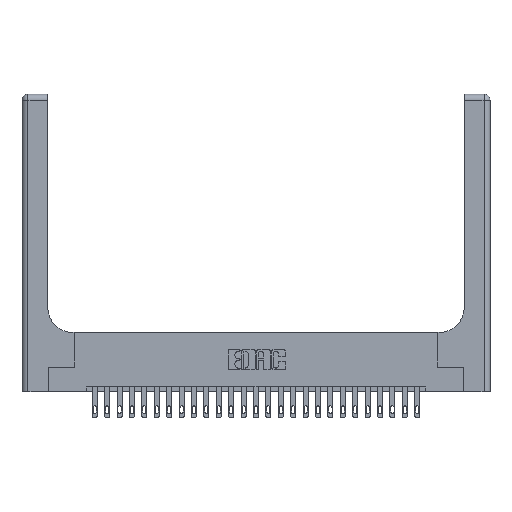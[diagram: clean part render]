
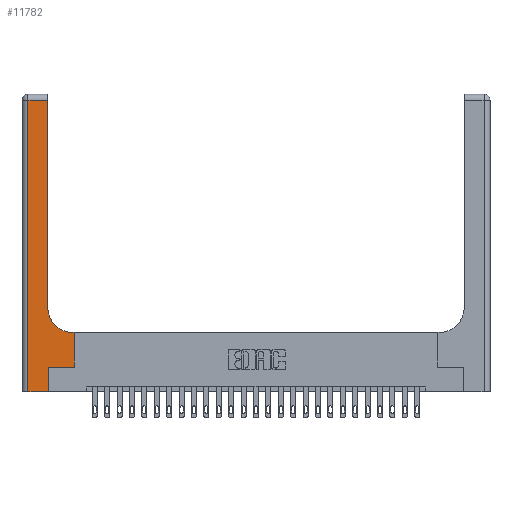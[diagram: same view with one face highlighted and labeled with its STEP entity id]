
A CAD part, top view. The second image highlights one B-rep face of the part: STEP entity #11782.
In plain terms, the highlighted planar face has unit normal (0, 0, 1).
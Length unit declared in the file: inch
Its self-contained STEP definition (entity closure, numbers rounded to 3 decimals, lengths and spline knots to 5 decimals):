
#100 = CARTESIAN_POINT ( 'NONE',  ( 0.265, 0.25, 0.37 ) ) ;
#306 = VERTEX_POINT ( 'NONE', #9878 ) ;
#396 = DIRECTION ( 'NONE',  ( -1., 0., 0. ) ) ;
#822 = EDGE_CURVE ( 'NONE', #2978, #306, #2323, .T. ) ;
#883 = EDGE_CURVE ( 'NONE', #9400, #15759, #10609, .T. ) ;
#951 = VERTEX_POINT ( 'NONE', #8666 ) ;
#962 = CARTESIAN_POINT ( 'NONE',  ( 0.528, 0.25, 0.37 ) ) ;
#973 = ORIENTED_EDGE ( 'NONE', *, *, #19436, .T. ) ;
#1063 = CARTESIAN_POINT ( 'NONE',  ( 0.26, 3., 0.37 ) ) ;
#1588 = ORIENTED_EDGE ( 'NONE', *, *, #12216, .T. ) ;
#2149 = LINE ( 'NONE', #100, #3455 ) ;
#2323 = LINE ( 'NONE', #17898, #21534 ) ;
#2620 = DIRECTION ( 'NONE',  ( 1., 0., 0. ) ) ;
#2686 = DIRECTION ( 'NONE',  ( -1., 0., 0. ) ) ;
#2876 = DIRECTION ( 'NONE',  ( 0., 0., -1. ) ) ;
#2966 = LINE ( 'NONE', #24124, #14047 ) ;
#2978 = VERTEX_POINT ( 'NONE', #19325 ) ;
#2990 = CARTESIAN_POINT ( 'NONE',  ( 0.26, 2.94, 0.37 ) ) ;
#3455 = VECTOR ( 'NONE', #5693, 39.37008 ) ;
#3918 = LINE ( 'NONE', #20876, #16368 ) ;
#4444 = PLANE ( 'NONE',  #10318 ) ;
#4510 = AXIS2_PLACEMENT_3D ( 'NONE', #6941, #2876, #2620 ) ;
#5407 = EDGE_CURVE ( 'NONE', #14916, #2978, #2966, .T. ) ;
#5564 = ORIENTED_EDGE ( 'NONE', *, *, #10845, .T. ) ;
#5693 = DIRECTION ( 'NONE',  ( 1., 0., 0. ) ) ;
#6185 = VERTEX_POINT ( 'NONE', #16670 ) ;
#6941 = CARTESIAN_POINT ( 'NONE',  ( 0.51, 0.85, 0.37 ) ) ;
#7314 = DIRECTION ( 'NONE',  ( -1., 0., 0. ) ) ;
#7535 = EDGE_LOOP ( 'NONE', ( #20932, #19525, #973, #1588, #21497, #5564, #16165, #24345, #13687 ) ) ;
#8648 = DIRECTION ( 'NONE',  ( 0., 0., -1. ) ) ;
#8666 = CARTESIAN_POINT ( 'NONE',  ( 0.26, 0.85, 0.37 ) ) ;
#9351 = LINE ( 'NONE', #1063, #21465 ) ;
#9400 = VERTEX_POINT ( 'NONE', #25192 ) ;
#9878 = CARTESIAN_POINT ( 'NONE',  ( 0.51, 0.6, 0.37 ) ) ;
#10318 = AXIS2_PLACEMENT_3D ( 'NONE', #10586, #8648, #2686 ) ;
#10497 = DIRECTION ( 'NONE',  ( 0., 1., 0. ) ) ;
#10586 = CARTESIAN_POINT ( 'NONE',  ( 0., 3., 0.37 ) ) ;
#10609 = LINE ( 'NONE', #12388, #12581 ) ;
#10845 = EDGE_CURVE ( 'NONE', #15759, #14916, #2149, .T. ) ;
#11064 = EDGE_CURVE ( 'NONE', #24900, #17267, #17045, .T. ) ;
#11662 = VECTOR ( 'NONE', #7314, 39.37008 ) ;
#11782 = ADVANCED_FACE ( 'NONE', ( #23973 ), #4444, .F. ) ;
#12216 = EDGE_CURVE ( 'NONE', #6185, #9400, #12340, .T. ) ;
#12340 = LINE ( 'NONE', #18346, #22368 ) ;
#12388 = CARTESIAN_POINT ( 'NONE',  ( 0.265, 0., 0.37 ) ) ;
#12581 = VECTOR ( 'NONE', #18397, 39.37008 ) ;
#13549 = EDGE_CURVE ( 'NONE', #951, #24900, #9351, .T. ) ;
#13687 = ORIENTED_EDGE ( 'NONE', *, *, #18368, .T. ) ;
#14047 = VECTOR ( 'NONE', #10497, 39.37008 ) ;
#14916 = VERTEX_POINT ( 'NONE', #962 ) ;
#15759 = VERTEX_POINT ( 'NONE', #20645 ) ;
#16165 = ORIENTED_EDGE ( 'NONE', *, *, #5407, .T. ) ;
#16368 = VECTOR ( 'NONE', #19337, 39.37008 ) ;
#16670 = CARTESIAN_POINT ( 'NONE',  ( 0.06, 0., 0.37 ) ) ;
#17045 = LINE ( 'NONE', #17291, #11662 ) ;
#17267 = VERTEX_POINT ( 'NONE', #18225 ) ;
#17291 = CARTESIAN_POINT ( 'NONE',  ( 0., 2.94, 0.37 ) ) ;
#17898 = CARTESIAN_POINT ( 'NONE',  ( 0.26, 0.6, 0.37 ) ) ;
#18225 = CARTESIAN_POINT ( 'NONE',  ( 0.06, 2.94, 0.37 ) ) ;
#18346 = CARTESIAN_POINT ( 'NONE',  ( 0., 0., 0.37 ) ) ;
#18368 = EDGE_CURVE ( 'NONE', #306, #951, #18379, .T. ) ;
#18379 = CIRCLE ( 'NONE', #4510, 0.25 ) ;
#18397 = DIRECTION ( 'NONE',  ( 0., 1., 0. ) ) ;
#19325 = CARTESIAN_POINT ( 'NONE',  ( 0.528, 0.6, 0.37 ) ) ;
#19337 = DIRECTION ( 'NONE',  ( 0., -1., 0. ) ) ;
#19436 = EDGE_CURVE ( 'NONE', #17267, #6185, #3918, .T. ) ;
#19525 = ORIENTED_EDGE ( 'NONE', *, *, #11064, .T. ) ;
#20109 = DIRECTION ( 'NONE',  ( 1., 0., 0. ) ) ;
#20645 = CARTESIAN_POINT ( 'NONE',  ( 0.265, 0.25, 0.37 ) ) ;
#20826 = DIRECTION ( 'NONE',  ( 0., 1., 0. ) ) ;
#20876 = CARTESIAN_POINT ( 'NONE',  ( 0.06, 3., 0.37 ) ) ;
#20932 = ORIENTED_EDGE ( 'NONE', *, *, #13549, .T. ) ;
#21465 = VECTOR ( 'NONE', #20826, 39.37008 ) ;
#21497 = ORIENTED_EDGE ( 'NONE', *, *, #883, .T. ) ;
#21534 = VECTOR ( 'NONE', #396, 39.37008 ) ;
#22368 = VECTOR ( 'NONE', #20109, 39.37008 ) ;
#23973 = FACE_OUTER_BOUND ( 'NONE', #7535, .T. ) ;
#24124 = CARTESIAN_POINT ( 'NONE',  ( 0.528, 0.25, 0.37 ) ) ;
#24345 = ORIENTED_EDGE ( 'NONE', *, *, #822, .T. ) ;
#24900 = VERTEX_POINT ( 'NONE', #2990 ) ;
#25192 = CARTESIAN_POINT ( 'NONE',  ( 0.265, 0., 0.37 ) ) ;
